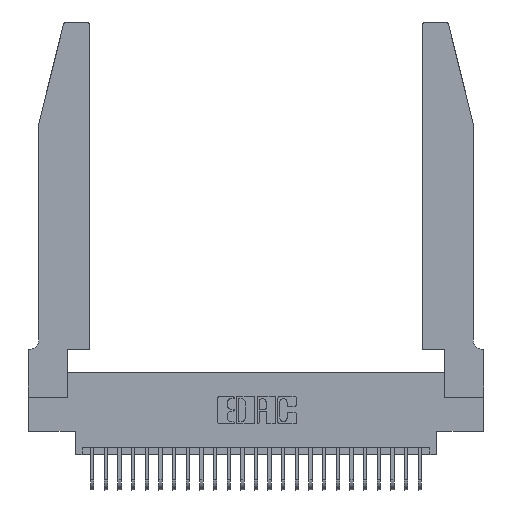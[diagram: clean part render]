
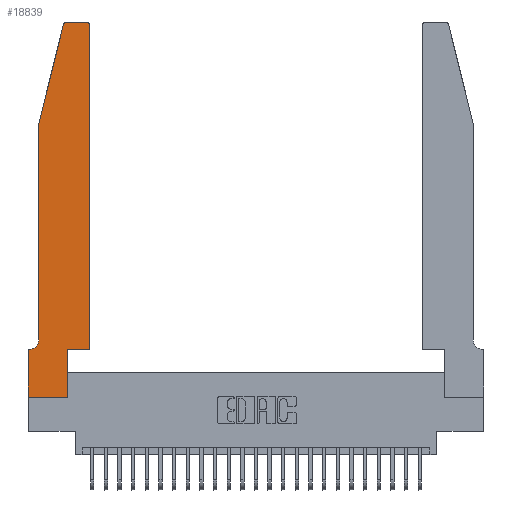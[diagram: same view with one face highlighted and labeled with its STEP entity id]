
A CAD part, top view. The second image highlights one B-rep face of the part: STEP entity #18839.
In plain terms, the highlighted planar face has unit normal (0, 0, 1).
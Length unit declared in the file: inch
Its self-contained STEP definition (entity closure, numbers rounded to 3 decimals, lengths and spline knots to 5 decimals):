
#72 = CARTESIAN_POINT ( 'NONE',  ( 0.4505, 2.72, 0.37 ) ) ;
#269 = CARTESIAN_POINT ( 'NONE',  ( 0.0055, 0.42, 0.37 ) ) ;
#455 = ORIENTED_EDGE ( 'NONE', *, *, #27454, .T. ) ;
#677 = CARTESIAN_POINT ( 'NONE',  ( 0.2865, 0.35, 0.37 ) ) ;
#1033 = VECTOR ( 'NONE', #1332, 39.37008 ) ;
#1332 = DIRECTION ( 'NONE',  ( 1., 0., 0. ) ) ;
#1417 = CIRCLE ( 'NONE', #7116, 0.07 ) ;
#1583 = CARTESIAN_POINT ( 'NONE',  ( 0.2865, 0.35, 0.37 ) ) ;
#1934 = DIRECTION ( 'NONE',  ( 1., 0., 0. ) ) ;
#2896 = CARTESIAN_POINT ( 'NONE',  ( 0.4505, 0.35, 0.37 ) ) ;
#3793 = ORIENTED_EDGE ( 'NONE', *, *, #16720, .T. ) ;
#3865 = PLANE ( 'NONE',  #15413 ) ;
#3902 = AXIS2_PLACEMENT_3D ( 'NONE', #15294, #6349, #19698 ) ;
#4795 = VECTOR ( 'NONE', #13269, 39.37008 ) ;
#6269 = ORIENTED_EDGE ( 'NONE', *, *, #14359, .T. ) ;
#6332 = ORIENTED_EDGE ( 'NONE', *, *, #18005, .T. ) ;
#6349 = DIRECTION ( 'NONE',  ( 0., 0., 1. ) ) ;
#6720 = CARTESIAN_POINT ( 'NONE',  ( 0.2605, 2.75, 0.37 ) ) ;
#6792 = VECTOR ( 'NONE', #18921, 39.37008 ) ;
#7044 = EDGE_CURVE ( 'NONE', #26928, #24993, #9175, .T. ) ;
#7095 = CARTESIAN_POINT ( 'NONE',  ( 0.0755, 2., 0.37 ) ) ;
#7116 = AXIS2_PLACEMENT_3D ( 'NONE', #269, #22025, #22127 ) ;
#7201 = CARTESIAN_POINT ( 'NONE',  ( 0., 0., 0.37 ) ) ;
#7202 = LINE ( 'NONE', #14491, #1033 ) ;
#7474 = LINE ( 'NONE', #15118, #22214 ) ;
#7914 = ORIENTED_EDGE ( 'NONE', *, *, #13515, .T. ) ;
#8131 = LINE ( 'NONE', #27157, #10910 ) ;
#8433 = VERTEX_POINT ( 'NONE', #19120 ) ;
#8531 = CARTESIAN_POINT ( 'NONE',  ( 0., 0.35, 0.37 ) ) ;
#8682 = LINE ( 'NONE', #6720, #19998 ) ;
#9023 = ORIENTED_EDGE ( 'NONE', *, *, #14587, .T. ) ;
#9131 = VERTEX_POINT ( 'NONE', #17703 ) ;
#9175 = LINE ( 'NONE', #23012, #6792 ) ;
#10296 = ORIENTED_EDGE ( 'NONE', *, *, #22717, .T. ) ;
#10372 = DIRECTION ( 'NONE',  ( 1., 0., 0. ) ) ;
#10563 = DIRECTION ( 'NONE',  ( 0., -1., 0. ) ) ;
#10703 = VECTOR ( 'NONE', #24691, 39.37008 ) ;
#10910 = VECTOR ( 'NONE', #14286, 39.37008 ) ;
#11502 = EDGE_CURVE ( 'NONE', #20438, #19625, #11714, .T. ) ;
#11714 = LINE ( 'NONE', #24965, #10703 ) ;
#12697 = VECTOR ( 'NONE', #10563, 39.37008 ) ;
#12772 = VERTEX_POINT ( 'NONE', #677 ) ;
#13239 = EDGE_CURVE ( 'NONE', #8433, #9131, #20566, .T. ) ;
#13269 = DIRECTION ( 'NONE',  ( -0.239, -0.971, 0. ) ) ;
#13515 = EDGE_CURVE ( 'NONE', #26025, #12772, #15768, .T. ) ;
#14161 = DIRECTION ( 'NONE',  ( 1., 0., 0. ) ) ;
#14286 = DIRECTION ( 'NONE',  ( 0., -1., 0. ) ) ;
#14352 = FACE_OUTER_BOUND ( 'NONE', #24541, .T. ) ;
#14359 = EDGE_CURVE ( 'NONE', #18040, #26025, #7474, .T. ) ;
#14491 = CARTESIAN_POINT ( 'NONE',  ( 0.4505, 0.35, 0.37 ) ) ;
#14587 = EDGE_CURVE ( 'NONE', #24993, #18040, #8131, .T. ) ;
#14762 = ORIENTED_EDGE ( 'NONE', *, *, #22035, .T. ) ;
#15118 = CARTESIAN_POINT ( 'NONE',  ( 0., 0., 0.37 ) ) ;
#15294 = CARTESIAN_POINT ( 'NONE',  ( 0.4205, 2.72, 0.37 ) ) ;
#15382 = DIRECTION ( 'NONE',  ( -1., 0., 0. ) ) ;
#15413 = AXIS2_PLACEMENT_3D ( 'NONE', #8531, #25924, #10372 ) ;
#15768 = LINE ( 'NONE', #1583, #23293 ) ;
#16082 = CARTESIAN_POINT ( 'NONE',  ( 0.4205, 2.75, 0.37 ) ) ;
#16720 = EDGE_CURVE ( 'NONE', #23481, #25957, #23691, .T. ) ;
#17032 = DIRECTION ( 'NONE',  ( 0., 1., 0. ) ) ;
#17101 = ORIENTED_EDGE ( 'NONE', *, *, #25990, .T. ) ;
#17703 = CARTESIAN_POINT ( 'NONE',  ( 0.0755, 0.42, 0.37 ) ) ;
#18005 = EDGE_CURVE ( 'NONE', #25957, #8433, #20901, .T. ) ;
#18040 = VERTEX_POINT ( 'NONE', #7201 ) ;
#18477 = CARTESIAN_POINT ( 'NONE',  ( 0.284, 2.72, 0.37 ) ) ;
#18666 = ORIENTED_EDGE ( 'NONE', *, *, #13239, .T. ) ;
#18839 = ADVANCED_FACE ( 'NONE', ( #14352 ), #3865, .T. ) ;
#18921 = DIRECTION ( 'NONE',  ( -1., 0., 0. ) ) ;
#19120 = CARTESIAN_POINT ( 'NONE',  ( 0.0755, 2., 0.37 ) ) ;
#19625 = VERTEX_POINT ( 'NONE', #72 ) ;
#19680 = CARTESIAN_POINT ( 'NONE',  ( 0.0755, 2., 0.37 ) ) ;
#19698 = DIRECTION ( 'NONE',  ( 1., 0., 0. ) ) ;
#19998 = VECTOR ( 'NONE', #15382, 39.37008 ) ;
#20438 = VERTEX_POINT ( 'NONE', #2896 ) ;
#20566 = LINE ( 'NONE', #19680, #12697 ) ;
#20901 = LINE ( 'NONE', #7095, #4795 ) ;
#22025 = DIRECTION ( 'NONE',  ( 0., 0., -1. ) ) ;
#22035 = EDGE_CURVE ( 'NONE', #26583, #23481, #8682, .T. ) ;
#22127 = DIRECTION ( 'NONE',  ( -1., 0., 0. ) ) ;
#22214 = VECTOR ( 'NONE', #1934, 39.37008 ) ;
#22218 = CIRCLE ( 'NONE', #3902, 0.03 ) ;
#22664 = CARTESIAN_POINT ( 'NONE',  ( 0.284, 2.75, 0.37 ) ) ;
#22717 = EDGE_CURVE ( 'NONE', #9131, #26928, #1417, .T. ) ;
#23012 = CARTESIAN_POINT ( 'NONE',  ( 0.0755, 0.35, 0.37 ) ) ;
#23293 = VECTOR ( 'NONE', #17032, 39.37008 ) ;
#23481 = VERTEX_POINT ( 'NONE', #22664 ) ;
#23691 = CIRCLE ( 'NONE', #26974, 0.03 ) ;
#23906 = CARTESIAN_POINT ( 'NONE',  ( 0., 0.35, 0.37 ) ) ;
#24169 = CARTESIAN_POINT ( 'NONE',  ( 0.0055, 0.35, 0.37 ) ) ;
#24541 = EDGE_LOOP ( 'NONE', ( #14762, #3793, #6332, #18666, #10296, #26939, #9023, #6269, #7914, #17101, #24835, #455 ) ) ;
#24691 = DIRECTION ( 'NONE',  ( 0., 1., 0. ) ) ;
#24835 = ORIENTED_EDGE ( 'NONE', *, *, #11502, .T. ) ;
#24965 = CARTESIAN_POINT ( 'NONE',  ( 0.4505, 0.35, 0.37 ) ) ;
#24993 = VERTEX_POINT ( 'NONE', #23906 ) ;
#25213 = CARTESIAN_POINT ( 'NONE',  ( 0.2865, 0., 0.37 ) ) ;
#25307 = CARTESIAN_POINT ( 'NONE',  ( 0.25487, 2.72718, 0.37 ) ) ;
#25924 = DIRECTION ( 'NONE',  ( 0., 0., 1. ) ) ;
#25957 = VERTEX_POINT ( 'NONE', #25307 ) ;
#25990 = EDGE_CURVE ( 'NONE', #12772, #20438, #7202, .T. ) ;
#26025 = VERTEX_POINT ( 'NONE', #25213 ) ;
#26583 = VERTEX_POINT ( 'NONE', #16082 ) ;
#26928 = VERTEX_POINT ( 'NONE', #24169 ) ;
#26939 = ORIENTED_EDGE ( 'NONE', *, *, #7044, .T. ) ;
#26974 = AXIS2_PLACEMENT_3D ( 'NONE', #18477, #27326, #14161 ) ;
#27157 = CARTESIAN_POINT ( 'NONE',  ( 0., 0., 0.37 ) ) ;
#27326 = DIRECTION ( 'NONE',  ( 0., 0., 1. ) ) ;
#27454 = EDGE_CURVE ( 'NONE', #19625, #26583, #22218, .T. ) ;
